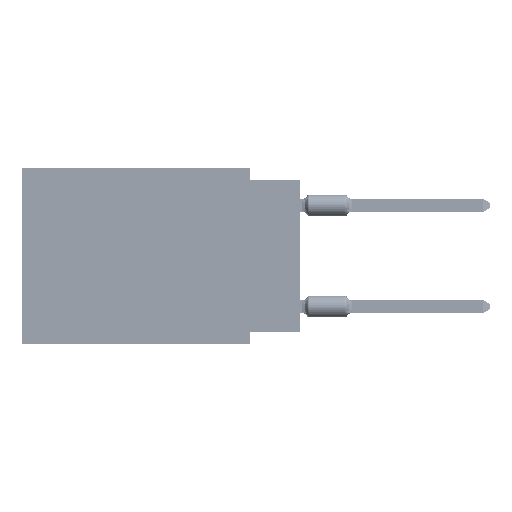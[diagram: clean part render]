
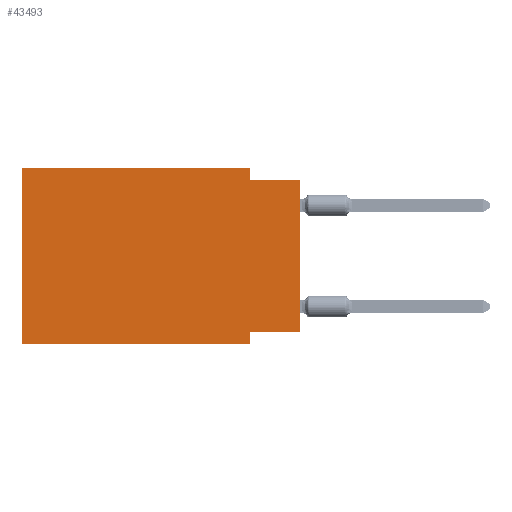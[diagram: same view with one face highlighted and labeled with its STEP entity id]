
A CAD part, left-side view. The second image highlights one B-rep face of the part: STEP entity #43493.
In plain terms, the highlighted planar face has unit normal (-1, 0, 0).
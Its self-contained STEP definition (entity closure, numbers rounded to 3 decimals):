
#2 = LINE ( 'NONE', #54355, #45079 ) ;
#538 = ORIENTED_EDGE ( 'NONE', *, *, #42536, .F. ) ;
#1318 = DIRECTION ( 'NONE',  ( 0., -1., 0. ) ) ;
#3973 = CARTESIAN_POINT ( 'NONE',  ( 0., 2.54, -8.89 ) ) ;
#4464 = VECTOR ( 'NONE', #52044, 1000. ) ;
#4544 = CARTESIAN_POINT ( 'NONE',  ( 0., 13.97, 0. ) ) ;
#6087 = EDGE_CURVE ( 'NONE', #7346, #28824, #2, .T. ) ;
#6387 = LINE ( 'NONE', #59203, #38269 ) ;
#7092 = ORIENTED_EDGE ( 'NONE', *, *, #47442, .F. ) ;
#7346 = VERTEX_POINT ( 'NONE', #72331 ) ;
#9561 = CARTESIAN_POINT ( 'NONE',  ( 0., 0., -0.635 ) ) ;
#13080 = VECTOR ( 'NONE', #57948, 1000. ) ;
#14087 = VERTEX_POINT ( 'NONE', #27806 ) ;
#15529 = CARTESIAN_POINT ( 'NONE',  ( 0., 0., -8.255 ) ) ;
#16248 = EDGE_LOOP ( 'NONE', ( #17762, #47613, #45433, #69876, #538, #54717, #7092, #60573 ) ) ;
#16519 = CARTESIAN_POINT ( 'NONE',  ( 0., 0., -0.635 ) ) ;
#17762 = ORIENTED_EDGE ( 'NONE', *, *, #20481, .T. ) ;
#20481 = EDGE_CURVE ( 'NONE', #66861, #32467, #30168, .T. ) ;
#27806 = CARTESIAN_POINT ( 'NONE',  ( 0., 2.54, -0.635 ) ) ;
#28274 = LINE ( 'NONE', #76676, #74296 ) ;
#28824 = VERTEX_POINT ( 'NONE', #31114 ) ;
#29028 = DIRECTION ( 'NONE',  ( 0., 0., -1. ) ) ;
#29381 = DIRECTION ( 'NONE',  ( 0., 0., 1. ) ) ;
#29491 = PLANE ( 'NONE',  #50297 ) ;
#30168 = LINE ( 'NONE', #59551, #48991 ) ;
#31114 = CARTESIAN_POINT ( 'NONE',  ( 0., 2.54, 0. ) ) ;
#32467 = VERTEX_POINT ( 'NONE', #9561 ) ;
#34669 = VECTOR ( 'NONE', #40737, 1000. ) ;
#38269 = VECTOR ( 'NONE', #29028, 1000. ) ;
#39347 = EDGE_CURVE ( 'NONE', #14087, #32467, #46704, .T. ) ;
#40737 = DIRECTION ( 'NONE',  ( 0., -1., 0. ) ) ;
#41373 = DIRECTION ( 'NONE',  ( 0., 0., 1. ) ) ;
#41614 = CARTESIAN_POINT ( 'NONE',  ( 0., 0., -8.255 ) ) ;
#42536 = EDGE_CURVE ( 'NONE', #58488, #7346, #28274, .T. ) ;
#43493 = ADVANCED_FACE ( 'NONE', ( #64825 ), #29491, .F. ) ;
#44552 = LINE ( 'NONE', #56463, #66940 ) ;
#45079 = VECTOR ( 'NONE', #59909, 1000. ) ;
#45433 = ORIENTED_EDGE ( 'NONE', *, *, #59138, .F. ) ;
#45445 = CARTESIAN_POINT ( 'NONE',  ( 0., 2.54, -8.255 ) ) ;
#46031 = LINE ( 'NONE', #3973, #13080 ) ;
#46562 = CARTESIAN_POINT ( 'NONE',  ( 0., 13.97, -8.89 ) ) ;
#46704 = LINE ( 'NONE', #16519, #34669 ) ;
#47442 = EDGE_CURVE ( 'NONE', #53076, #54424, #46031, .T. ) ;
#47613 = ORIENTED_EDGE ( 'NONE', *, *, #39347, .F. ) ;
#48991 = VECTOR ( 'NONE', #29381, 1000. ) ;
#50297 = AXIS2_PLACEMENT_3D ( 'NONE', #4544, #71558, #52942 ) ;
#52044 = DIRECTION ( 'NONE',  ( 0., 1., 0. ) ) ;
#52942 = DIRECTION ( 'NONE',  ( 0., 0., -1. ) ) ;
#53076 = VERTEX_POINT ( 'NONE', #45445 ) ;
#53201 = EDGE_CURVE ( 'NONE', #58488, #54424, #44552, .T. ) ;
#54355 = CARTESIAN_POINT ( 'NONE',  ( 0., 13.97, 0. ) ) ;
#54424 = VERTEX_POINT ( 'NONE', #56477 ) ;
#54717 = ORIENTED_EDGE ( 'NONE', *, *, #53201, .T. ) ;
#56463 = CARTESIAN_POINT ( 'NONE',  ( 0., 13.97, -8.89 ) ) ;
#56477 = CARTESIAN_POINT ( 'NONE',  ( 0., 2.54, -8.89 ) ) ;
#56833 = LINE ( 'NONE', #15529, #4464 ) ;
#57948 = DIRECTION ( 'NONE',  ( 0., 0., -1. ) ) ;
#58488 = VERTEX_POINT ( 'NONE', #46562 ) ;
#59138 = EDGE_CURVE ( 'NONE', #28824, #14087, #6387, .T. ) ;
#59203 = CARTESIAN_POINT ( 'NONE',  ( 0., 2.54, 0. ) ) ;
#59551 = CARTESIAN_POINT ( 'NONE',  ( 0., 0., 0. ) ) ;
#59909 = DIRECTION ( 'NONE',  ( 0., -1., 0. ) ) ;
#60573 = ORIENTED_EDGE ( 'NONE', *, *, #63363, .F. ) ;
#63363 = EDGE_CURVE ( 'NONE', #66861, #53076, #56833, .T. ) ;
#64825 = FACE_OUTER_BOUND ( 'NONE', #16248, .T. ) ;
#66861 = VERTEX_POINT ( 'NONE', #41614 ) ;
#66940 = VECTOR ( 'NONE', #1318, 1000. ) ;
#69876 = ORIENTED_EDGE ( 'NONE', *, *, #6087, .F. ) ;
#71558 = DIRECTION ( 'NONE',  ( 1., 0., 0. ) ) ;
#72331 = CARTESIAN_POINT ( 'NONE',  ( 0., 13.97, 0. ) ) ;
#74296 = VECTOR ( 'NONE', #41373, 1000. ) ;
#76676 = CARTESIAN_POINT ( 'NONE',  ( 0., 13.97, 0. ) ) ;
